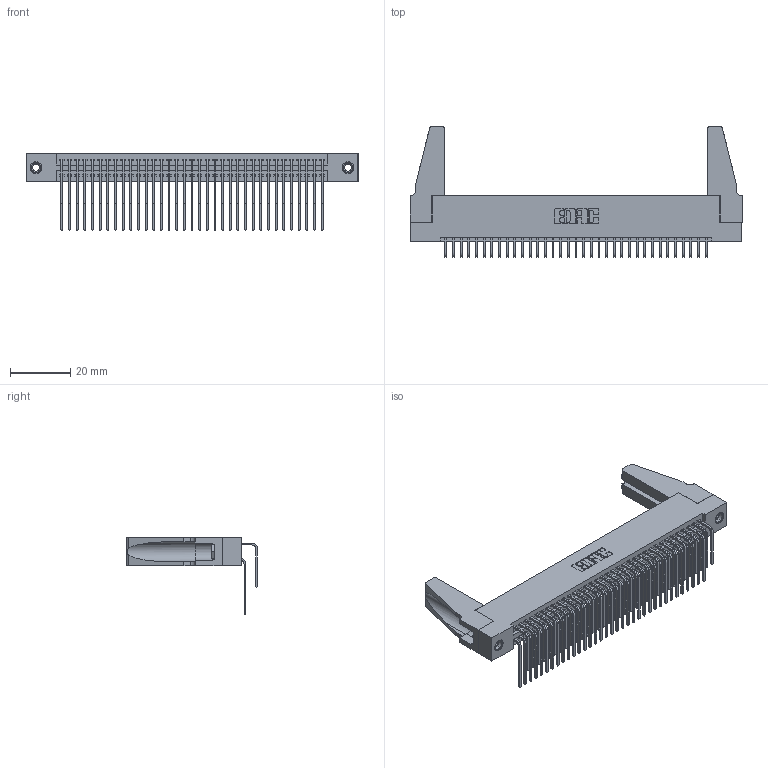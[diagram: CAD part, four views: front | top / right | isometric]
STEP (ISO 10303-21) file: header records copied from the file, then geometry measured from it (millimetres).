
FILE_DESCRIPTION (( 'STEP AP203' ), '1' );
FILE_NAME ('345-070-559-288.STEP', '2019-10-31T01:52:16', ( '' ), ( '' ), 'SwSTEP 2.0', 'SolidWorks 2016', '' );
FILE_SCHEMA (( 'CONFIG_CONTROL_DESIGN' ));
Length unit declared in the file: inch
Products named in the file (6): 345-292-001_559 Tail - 2; 345-070-559-288; 345-292-001_558 559 Tail - 1; 345 Part_Flush Mounting Lugs - 0.156 Dia-TH; 345-220-078_345-220-088; 345-250-001_345-250-001-102
Assembly tree (75 placements, depth 2):
  345-070-559-288
    345 Part_Flush Mounting Lugs - 0.156 Dia-TH
    345-292-001_558 559 Tail - 1  x35
    345-292-001_559 Tail - 2  x35
    345-250-001_345-250-001-102  x2
    345-220-078_345-220-088  x2
Bounding box: 110.13 x 43.42 x 25.53 mm (x, y, z)
Volume: 14289.8 mm3; surface area: 21200.5 mm2
Topology: 75 solids, 75 shells, 3890 faces, 11505 edges, 7566 vertices
Faces by surface type: plane 2602, cylinder 1272, cone 12, torus 4
Entity records: 32204 total; most frequent: CARTESIAN_POINT 5445, ORIENTED_EDGE 5288, DIRECTION 4788, EDGE_CURVE 2644, VECTOR 2290, LINE 2290, VERTEX_POINT 1754, AXIS2_PLACEMENT_3D 1249
